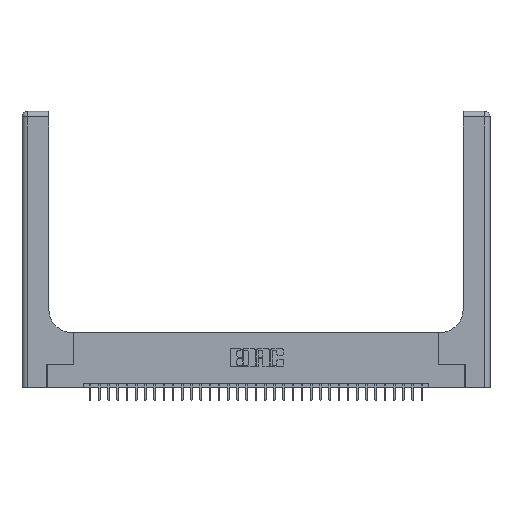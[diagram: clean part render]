
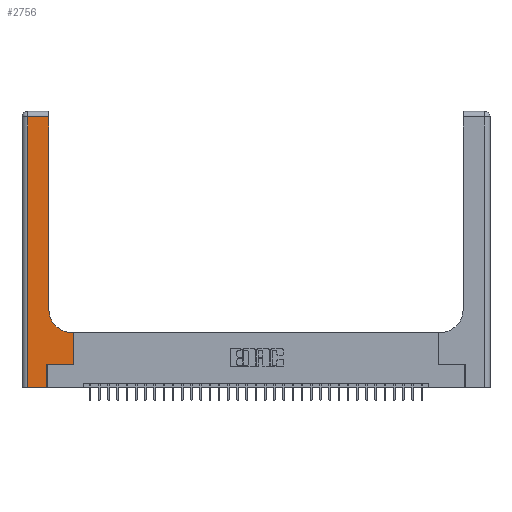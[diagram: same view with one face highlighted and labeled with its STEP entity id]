
A CAD part, top view. The second image highlights one B-rep face of the part: STEP entity #2756.
In plain terms, the highlighted planar face has unit normal (0, 0, 1).
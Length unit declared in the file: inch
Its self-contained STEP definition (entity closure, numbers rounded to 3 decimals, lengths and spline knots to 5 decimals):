
#297 = ORIENTED_EDGE ( 'NONE', *, *, #33650, .T. ) ;
#495 = CARTESIAN_POINT ( 'NONE',  ( 0.5415, 0.85, 0.37 ) ) ;
#631 = CARTESIAN_POINT ( 'NONE',  ( 0.5415, 0.6, 0.37 ) ) ;
#638 = LINE ( 'NONE', #11781, #26336 ) ;
#980 = ORIENTED_EDGE ( 'NONE', *, *, #19082, .T. ) ;
#1029 = VECTOR ( 'NONE', #11017, 39.37008 ) ;
#1286 = VERTEX_POINT ( 'NONE', #16656 ) ;
#1613 = LINE ( 'NONE', #34018, #13127 ) ;
#2756 = ADVANCED_FACE ( 'NONE', ( #17761 ), #9631, .F. ) ;
#3179 = ORIENTED_EDGE ( 'NONE', *, *, #27769, .T. ) ;
#3813 = VERTEX_POINT ( 'NONE', #30177 ) ;
#4155 = CARTESIAN_POINT ( 'NONE',  ( 0.269, 0., 0.37 ) ) ;
#4158 = EDGE_CURVE ( 'NONE', #5532, #15166, #27464, .T. ) ;
#4454 = DIRECTION ( 'NONE',  ( 1., 0., 0. ) ) ;
#4723 = VERTEX_POINT ( 'NONE', #6550 ) ;
#5137 = VECTOR ( 'NONE', #15295, 39.37008 ) ;
#5227 = VECTOR ( 'NONE', #15893, 39.37008 ) ;
#5372 = DIRECTION ( 'NONE',  ( 1., 0., 0. ) ) ;
#5532 = VERTEX_POINT ( 'NONE', #33375 ) ;
#5721 = CARTESIAN_POINT ( 'NONE',  ( 0., 2.94, 0.37 ) ) ;
#6327 = AXIS2_PLACEMENT_3D ( 'NONE', #495, #7968, #8493 ) ;
#6550 = CARTESIAN_POINT ( 'NONE',  ( 0.5585, 0.25, 0.37 ) ) ;
#6634 = CARTESIAN_POINT ( 'NONE',  ( 0., 3., 0.37 ) ) ;
#6802 = DIRECTION ( 'NONE',  ( 0., -1., 0. ) ) ;
#7092 = VECTOR ( 'NONE', #5372, 39.37008 ) ;
#7181 = LINE ( 'NONE', #4155, #5137 ) ;
#7863 = ORIENTED_EDGE ( 'NONE', *, *, #17815, .T. ) ;
#7968 = DIRECTION ( 'NONE',  ( 0., 0., -1. ) ) ;
#8231 = CARTESIAN_POINT ( 'NONE',  ( 0.2915, 0.6, 0.37 ) ) ;
#8413 = DIRECTION ( 'NONE',  ( -1., 0., 0. ) ) ;
#8493 = DIRECTION ( 'NONE',  ( 1., 0., 0. ) ) ;
#8724 = EDGE_CURVE ( 'NONE', #10545, #20448, #7181, .T. ) ;
#9357 = EDGE_CURVE ( 'NONE', #31904, #3813, #10266, .T. ) ;
#9631 = PLANE ( 'NONE',  #31516 ) ;
#9941 = CARTESIAN_POINT ( 'NONE',  ( 0.06, 2.94, 0.37 ) ) ;
#10266 = CIRCLE ( 'NONE', #6327, 0.25 ) ;
#10545 = VERTEX_POINT ( 'NONE', #29780 ) ;
#10592 = CARTESIAN_POINT ( 'NONE',  ( 0.2915, 3., 0.37 ) ) ;
#11017 = DIRECTION ( 'NONE',  ( -1., 0., 0. ) ) ;
#11781 = CARTESIAN_POINT ( 'NONE',  ( 0.5585, 0.25, 0.37 ) ) ;
#12148 = CARTESIAN_POINT ( 'NONE',  ( 0.5585, 0.6, 0.37 ) ) ;
#12613 = EDGE_CURVE ( 'NONE', #3813, #5532, #25821, .T. ) ;
#13127 = VECTOR ( 'NONE', #4454, 39.37008 ) ;
#15166 = VERTEX_POINT ( 'NONE', #9941 ) ;
#15295 = DIRECTION ( 'NONE',  ( 0., 1., 0. ) ) ;
#15454 = CARTESIAN_POINT ( 'NONE',  ( 0.269, 0.25, 0.37 ) ) ;
#15893 = DIRECTION ( 'NONE',  ( 0., 1., 0. ) ) ;
#16656 = CARTESIAN_POINT ( 'NONE',  ( 0.06, 0., 0.37 ) ) ;
#16718 = ORIENTED_EDGE ( 'NONE', *, *, #4158, .T. ) ;
#17234 = DIRECTION ( 'NONE',  ( 0., 0., -1. ) ) ;
#17627 = CARTESIAN_POINT ( 'NONE',  ( 0.269, 0.25, 0.37 ) ) ;
#17761 = FACE_OUTER_BOUND ( 'NONE', #23829, .T. ) ;
#17815 = EDGE_CURVE ( 'NONE', #20448, #4723, #18805, .T. ) ;
#18805 = LINE ( 'NONE', #15454, #7092 ) ;
#19082 = EDGE_CURVE ( 'NONE', #4723, #27870, #638, .T. ) ;
#19484 = VECTOR ( 'NONE', #6802, 39.37008 ) ;
#20033 = LINE ( 'NONE', #31043, #19484 ) ;
#20448 = VERTEX_POINT ( 'NONE', #17627 ) ;
#22576 = DIRECTION ( 'NONE',  ( 0., 1., 0. ) ) ;
#23829 = EDGE_LOOP ( 'NONE', ( #32197, #16718, #28312, #3179, #28461, #7863, #980, #297, #24029 ) ) ;
#24029 = ORIENTED_EDGE ( 'NONE', *, *, #9357, .T. ) ;
#24495 = LINE ( 'NONE', #8231, #30832 ) ;
#25821 = LINE ( 'NONE', #10592, #5227 ) ;
#26336 = VECTOR ( 'NONE', #22576, 39.37008 ) ;
#27464 = LINE ( 'NONE', #5721, #1029 ) ;
#27769 = EDGE_CURVE ( 'NONE', #1286, #10545, #1613, .T. ) ;
#27870 = VERTEX_POINT ( 'NONE', #12148 ) ;
#28312 = ORIENTED_EDGE ( 'NONE', *, *, #33871, .T. ) ;
#28461 = ORIENTED_EDGE ( 'NONE', *, *, #8724, .T. ) ;
#29780 = CARTESIAN_POINT ( 'NONE',  ( 0.269, 0., 0.37 ) ) ;
#30177 = CARTESIAN_POINT ( 'NONE',  ( 0.2915, 0.85, 0.37 ) ) ;
#30832 = VECTOR ( 'NONE', #8413, 39.37008 ) ;
#30872 = DIRECTION ( 'NONE',  ( -1., 0., 0. ) ) ;
#31043 = CARTESIAN_POINT ( 'NONE',  ( 0.06, 3., 0.37 ) ) ;
#31516 = AXIS2_PLACEMENT_3D ( 'NONE', #6634, #17234, #30872 ) ;
#31904 = VERTEX_POINT ( 'NONE', #631 ) ;
#32197 = ORIENTED_EDGE ( 'NONE', *, *, #12613, .T. ) ;
#33375 = CARTESIAN_POINT ( 'NONE',  ( 0.2915, 2.94, 0.37 ) ) ;
#33650 = EDGE_CURVE ( 'NONE', #27870, #31904, #24495, .T. ) ;
#33871 = EDGE_CURVE ( 'NONE', #15166, #1286, #20033, .T. ) ;
#34018 = CARTESIAN_POINT ( 'NONE',  ( 0., 0., 0.37 ) ) ;
